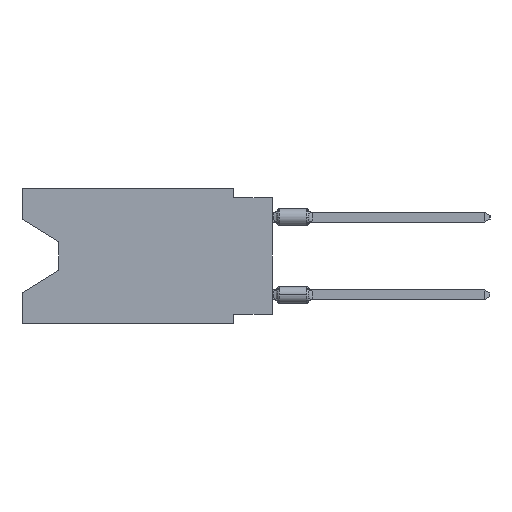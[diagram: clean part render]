
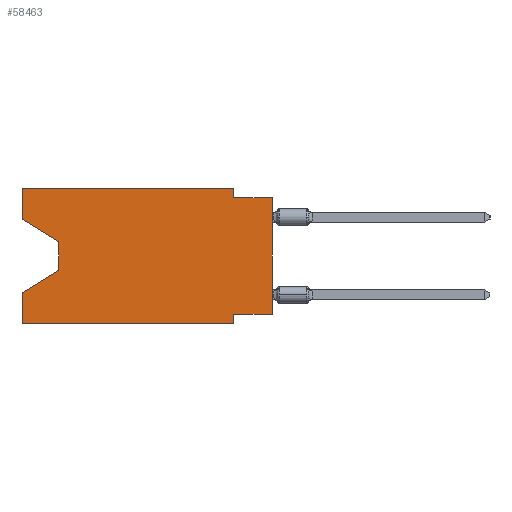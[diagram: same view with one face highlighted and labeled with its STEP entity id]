
A CAD part, left-side view. The second image highlights one B-rep face of the part: STEP entity #58463.
In plain terms, the highlighted planar face has unit normal (-1, 0, 0).
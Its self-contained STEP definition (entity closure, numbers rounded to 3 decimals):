
#522 = PLANE ( 'NONE',  #37000 ) ;
#740 = DIRECTION ( 'NONE',  ( 0., 1., 0. ) ) ;
#2965 = VECTOR ( 'NONE', #7552, 1000. ) ;
#3199 = LINE ( 'NONE', #21713, #11388 ) ;
#3375 = EDGE_CURVE ( 'NONE', #48185, #7377, #30083, .T. ) ;
#3506 = ORIENTED_EDGE ( 'NONE', *, *, #31812, .F. ) ;
#4239 = EDGE_CURVE ( 'NONE', #28399, #29868, #21204, .T. ) ;
#4367 = LINE ( 'NONE', #12183, #2965 ) ;
#4480 = CARTESIAN_POINT ( 'NONE',  ( 0., 13.97, -5.385 ) ) ;
#4753 = VERTEX_POINT ( 'NONE', #21884 ) ;
#5218 = CARTESIAN_POINT ( 'NONE',  ( 0., 13.97, -3.505 ) ) ;
#5505 = CARTESIAN_POINT ( 'NONE',  ( 0., 0., -8.255 ) ) ;
#6074 = DIRECTION ( 'NONE',  ( 1., 0., 0. ) ) ;
#7377 = VERTEX_POINT ( 'NONE', #58179 ) ;
#7535 = EDGE_CURVE ( 'NONE', #34691, #30594, #3199, .T. ) ;
#7552 = DIRECTION ( 'NONE',  ( 0., -1., 0. ) ) ;
#8162 = CARTESIAN_POINT ( 'NONE',  ( 0., 2.54, -8.255 ) ) ;
#8167 = ORIENTED_EDGE ( 'NONE', *, *, #7535, .F. ) ;
#8383 = ORIENTED_EDGE ( 'NONE', *, *, #4239, .F. ) ;
#9398 = EDGE_CURVE ( 'NONE', #40944, #29868, #26637, .T. ) ;
#9707 = CARTESIAN_POINT ( 'NONE',  ( 0., 0., 0. ) ) ;
#9781 = FACE_OUTER_BOUND ( 'NONE', #14743, .T. ) ;
#10087 = EDGE_CURVE ( 'NONE', #58367, #4753, #24075, .T. ) ;
#11388 = VECTOR ( 'NONE', #22026, 1000. ) ;
#11502 = ORIENTED_EDGE ( 'NONE', *, *, #36835, .F. ) ;
#12183 = CARTESIAN_POINT ( 'NONE',  ( 0., 0., -0.635 ) ) ;
#12328 = DIRECTION ( 'NONE',  ( 0., -1., 0. ) ) ;
#13487 = CARTESIAN_POINT ( 'NONE',  ( 0., 16.383, -6.852 ) ) ;
#13561 = ORIENTED_EDGE ( 'NONE', *, *, #9398, .T. ) ;
#14743 = EDGE_LOOP ( 'NONE', ( #17499, #33457, #13561, #8383, #60228, #44896, #24833, #31288, #3506, #8167, #11502, #38556 ) ) ;
#15232 = VECTOR ( 'NONE', #40034, 1000. ) ;
#16072 = LINE ( 'NONE', #29357, #38736 ) ;
#16497 = DIRECTION ( 'NONE',  ( 0., 0., -1. ) ) ;
#17499 = ORIENTED_EDGE ( 'NONE', *, *, #32419, .T. ) ;
#19260 = CARTESIAN_POINT ( 'NONE',  ( 0., 0., -0.635 ) ) ;
#19709 = DIRECTION ( 'NONE',  ( 0., -0.855, -0.519 ) ) ;
#20601 = VECTOR ( 'NONE', #42593, 1000. ) ;
#21204 = LINE ( 'NONE', #44063, #15232 ) ;
#21660 = VERTEX_POINT ( 'NONE', #19260 ) ;
#21713 = CARTESIAN_POINT ( 'NONE',  ( 0., 2.54, 0. ) ) ;
#21884 = CARTESIAN_POINT ( 'NONE',  ( 0., 16.383, 0. ) ) ;
#22026 = DIRECTION ( 'NONE',  ( 0., 0., -1. ) ) ;
#23062 = VECTOR ( 'NONE', #16497, 1000. ) ;
#24075 = LINE ( 'NONE', #60825, #20601 ) ;
#24833 = ORIENTED_EDGE ( 'NONE', *, *, #24892, .F. ) ;
#24892 = EDGE_CURVE ( 'NONE', #38370, #48185, #32835, .T. ) ;
#25002 = VECTOR ( 'NONE', #12328, 1000. ) ;
#26073 = CARTESIAN_POINT ( 'NONE',  ( 0., 2.54, 0. ) ) ;
#26087 = VERTEX_POINT ( 'NONE', #50620 ) ;
#26190 = EDGE_CURVE ( 'NONE', #26087, #40944, #47514, .T. ) ;
#26325 = VECTOR ( 'NONE', #740, 1000. ) ;
#26637 = LINE ( 'NONE', #32484, #38325 ) ;
#28399 = VERTEX_POINT ( 'NONE', #28740 ) ;
#28740 = CARTESIAN_POINT ( 'NONE',  ( 0., 16.383, -8.89 ) ) ;
#29357 = CARTESIAN_POINT ( 'NONE',  ( 0., 16.383, -8.89 ) ) ;
#29868 = VERTEX_POINT ( 'NONE', #13487 ) ;
#30083 = LINE ( 'NONE', #34119, #23062 ) ;
#30594 = VERTEX_POINT ( 'NONE', #43178 ) ;
#31288 = ORIENTED_EDGE ( 'NONE', *, *, #41051, .T. ) ;
#31359 = VECTOR ( 'NONE', #43344, 1000. ) ;
#31812 = EDGE_CURVE ( 'NONE', #30594, #21660, #4367, .T. ) ;
#32419 = EDGE_CURVE ( 'NONE', #58367, #26087, #33294, .T. ) ;
#32484 = CARTESIAN_POINT ( 'NONE',  ( 0., 13.97, -5.385 ) ) ;
#32835 = LINE ( 'NONE', #51682, #26325 ) ;
#33294 = LINE ( 'NONE', #42550, #39495 ) ;
#33457 = ORIENTED_EDGE ( 'NONE', *, *, #26190, .T. ) ;
#33855 = DIRECTION ( 'NONE',  ( 0., 0., -1. ) ) ;
#33999 = DIRECTION ( 'NONE',  ( 0., -1., 0. ) ) ;
#34101 = LINE ( 'NONE', #9707, #31359 ) ;
#34119 = CARTESIAN_POINT ( 'NONE',  ( 0., 2.54, -8.89 ) ) ;
#34691 = VERTEX_POINT ( 'NONE', #26073 ) ;
#36835 = EDGE_CURVE ( 'NONE', #4753, #34691, #54627, .T. ) ;
#37000 = AXIS2_PLACEMENT_3D ( 'NONE', #42804, #6074, #33855 ) ;
#38325 = VECTOR ( 'NONE', #55366, 1000. ) ;
#38370 = VERTEX_POINT ( 'NONE', #5505 ) ;
#38556 = ORIENTED_EDGE ( 'NONE', *, *, #10087, .F. ) ;
#38736 = VECTOR ( 'NONE', #33999, 1000. ) ;
#39495 = VECTOR ( 'NONE', #19709, 1000. ) ;
#40034 = DIRECTION ( 'NONE',  ( 0., 0., 1. ) ) ;
#40944 = VERTEX_POINT ( 'NONE', #4480 ) ;
#41051 = EDGE_CURVE ( 'NONE', #38370, #21660, #34101, .T. ) ;
#41932 = VECTOR ( 'NONE', #54188, 1000. ) ;
#42550 = CARTESIAN_POINT ( 'NONE',  ( 0., 16.383, -2.038 ) ) ;
#42593 = DIRECTION ( 'NONE',  ( 0., 0., 1. ) ) ;
#42804 = CARTESIAN_POINT ( 'NONE',  ( 0., 16.383, 0. ) ) ;
#43178 = CARTESIAN_POINT ( 'NONE',  ( 0., 2.54, -0.635 ) ) ;
#43344 = DIRECTION ( 'NONE',  ( 0., 0., 1. ) ) ;
#44063 = CARTESIAN_POINT ( 'NONE',  ( 0., 16.383, 0. ) ) ;
#44896 = ORIENTED_EDGE ( 'NONE', *, *, #3375, .F. ) ;
#47514 = LINE ( 'NONE', #5218, #41932 ) ;
#48185 = VERTEX_POINT ( 'NONE', #8162 ) ;
#50217 = EDGE_CURVE ( 'NONE', #28399, #7377, #16072, .T. ) ;
#50620 = CARTESIAN_POINT ( 'NONE',  ( 0., 13.97, -3.505 ) ) ;
#51472 = CARTESIAN_POINT ( 'NONE',  ( 0., 16.383, -2.038 ) ) ;
#51682 = CARTESIAN_POINT ( 'NONE',  ( 0., 0., -8.255 ) ) ;
#54017 = CARTESIAN_POINT ( 'NONE',  ( 0., 16.383, 0. ) ) ;
#54188 = DIRECTION ( 'NONE',  ( 0., 0., -1. ) ) ;
#54627 = LINE ( 'NONE', #54017, #25002 ) ;
#55366 = DIRECTION ( 'NONE',  ( 0., 0.855, -0.519 ) ) ;
#58179 = CARTESIAN_POINT ( 'NONE',  ( 0., 2.54, -8.89 ) ) ;
#58367 = VERTEX_POINT ( 'NONE', #51472 ) ;
#58463 = ADVANCED_FACE ( 'NONE', ( #9781 ), #522, .F. ) ;
#60228 = ORIENTED_EDGE ( 'NONE', *, *, #50217, .T. ) ;
#60825 = CARTESIAN_POINT ( 'NONE',  ( 0., 16.383, 0. ) ) ;
